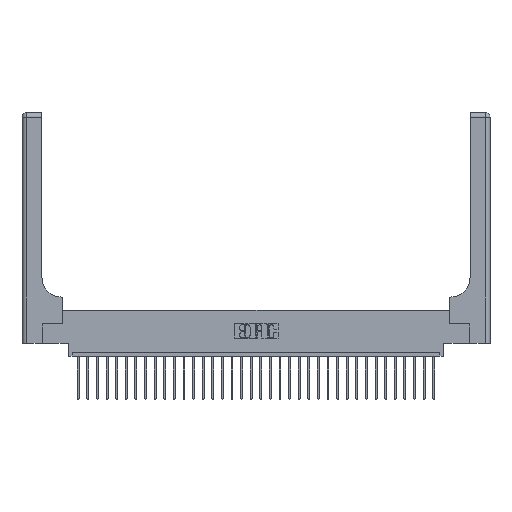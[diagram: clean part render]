
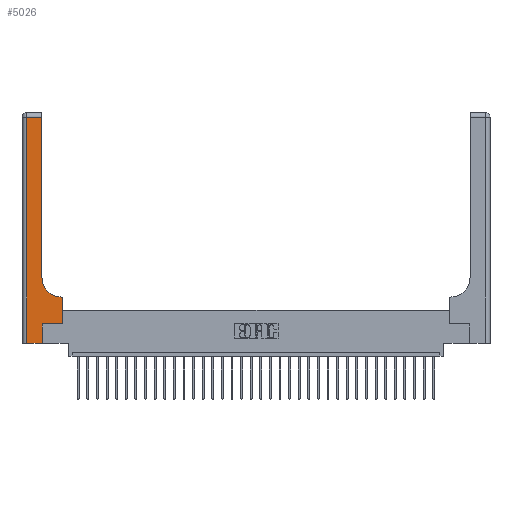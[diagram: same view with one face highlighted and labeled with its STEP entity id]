
A CAD part, top view. The second image highlights one B-rep face of the part: STEP entity #5026.
In plain terms, the highlighted planar face has unit normal (0, 0, 1).
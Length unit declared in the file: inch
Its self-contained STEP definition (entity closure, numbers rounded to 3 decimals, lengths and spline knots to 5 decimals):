
#54 = DIRECTION ( 'NONE',  ( -1., 0., 0. ) ) ;
#250 = CARTESIAN_POINT ( 'NONE',  ( 0.26, 2.94, 0.37 ) ) ;
#1270 = EDGE_LOOP ( 'NONE', ( #12998, #25585, #28772, #19783, #25614, #28763, #11897, #7678, #22462 ) ) ;
#1309 = DIRECTION ( 'NONE',  ( 0., -1., 0. ) ) ;
#1409 = EDGE_CURVE ( 'NONE', #23667, #22052, #14912, .T. ) ;
#2020 = VECTOR ( 'NONE', #9979, 39.37008 ) ;
#2103 = DIRECTION ( 'NONE',  ( 1., 0., 0. ) ) ;
#2382 = VECTOR ( 'NONE', #54, 39.37008 ) ;
#3548 = CIRCLE ( 'NONE', #27629, 0.25 ) ;
#3644 = VECTOR ( 'NONE', #27688, 39.37008 ) ;
#3798 = VECTOR ( 'NONE', #1309, 39.37008 ) ;
#4143 = VERTEX_POINT ( 'NONE', #25216 ) ;
#5026 = ADVANCED_FACE ( 'NONE', ( #11676 ), #18941, .F. ) ;
#5124 = DIRECTION ( 'NONE',  ( 0., 1., 0. ) ) ;
#6511 = DIRECTION ( 'NONE',  ( 1., 0., 0. ) ) ;
#7032 = VERTEX_POINT ( 'NONE', #24123 ) ;
#7678 = ORIENTED_EDGE ( 'NONE', *, *, #9285, .T. ) ;
#8913 = DIRECTION ( 'NONE',  ( 0., 0., -1. ) ) ;
#9285 = EDGE_CURVE ( 'NONE', #28783, #4143, #15762, .T. ) ;
#9369 = CARTESIAN_POINT ( 'NONE',  ( 0., 0., 0.37 ) ) ;
#9979 = DIRECTION ( 'NONE',  ( -1., 0., 0. ) ) ;
#10131 = VERTEX_POINT ( 'NONE', #18291 ) ;
#10431 = CARTESIAN_POINT ( 'NONE',  ( 0.528, 0.6, 0.37 ) ) ;
#10972 = VECTOR ( 'NONE', #6511, 39.37008 ) ;
#11676 = FACE_OUTER_BOUND ( 'NONE', #1270, .T. ) ;
#11800 = CARTESIAN_POINT ( 'NONE',  ( 0.06, 2.94, 0.37 ) ) ;
#11897 = ORIENTED_EDGE ( 'NONE', *, *, #12478, .T. ) ;
#12478 = EDGE_CURVE ( 'NONE', #27500, #28783, #18106, .T. ) ;
#12998 = ORIENTED_EDGE ( 'NONE', *, *, #15473, .T. ) ;
#14522 = CARTESIAN_POINT ( 'NONE',  ( 0.528, 0.25, 0.37 ) ) ;
#14668 = VECTOR ( 'NONE', #5124, 39.37008 ) ;
#14912 = LINE ( 'NONE', #20059, #3798 ) ;
#15473 = EDGE_CURVE ( 'NONE', #10131, #28225, #29435, .T. ) ;
#15762 = LINE ( 'NONE', #29845, #2382 ) ;
#15955 = EDGE_CURVE ( 'NONE', #4143, #10131, #3548, .T. ) ;
#16563 = VECTOR ( 'NONE', #22333, 39.37008 ) ;
#18106 = LINE ( 'NONE', #25066, #28516 ) ;
#18232 = CARTESIAN_POINT ( 'NONE',  ( 0.26, 3., 0.37 ) ) ;
#18291 = CARTESIAN_POINT ( 'NONE',  ( 0.26, 0.85, 0.37 ) ) ;
#18486 = CARTESIAN_POINT ( 'NONE',  ( 0., 3., 0.37 ) ) ;
#18571 = LINE ( 'NONE', #27647, #14668 ) ;
#18933 = VERTEX_POINT ( 'NONE', #20985 ) ;
#18941 = PLANE ( 'NONE',  #20073 ) ;
#19783 = ORIENTED_EDGE ( 'NONE', *, *, #28941, .T. ) ;
#20059 = CARTESIAN_POINT ( 'NONE',  ( 0.06, 3., 0.37 ) ) ;
#20073 = AXIS2_PLACEMENT_3D ( 'NONE', #18486, #28171, #27709 ) ;
#20985 = CARTESIAN_POINT ( 'NONE',  ( 0.265, 0.25, 0.37 ) ) ;
#21346 = EDGE_CURVE ( 'NONE', #28225, #23667, #24191, .T. ) ;
#22052 = VERTEX_POINT ( 'NONE', #28991 ) ;
#22333 = DIRECTION ( 'NONE',  ( 0., 1., 0. ) ) ;
#22462 = ORIENTED_EDGE ( 'NONE', *, *, #15955, .T. ) ;
#22979 = EDGE_CURVE ( 'NONE', #7032, #18933, #18571, .T. ) ;
#23174 = LINE ( 'NONE', #23764, #3644 ) ;
#23297 = LINE ( 'NONE', #9369, #10972 ) ;
#23667 = VERTEX_POINT ( 'NONE', #11800 ) ;
#23764 = CARTESIAN_POINT ( 'NONE',  ( 0.265, 0.25, 0.37 ) ) ;
#24123 = CARTESIAN_POINT ( 'NONE',  ( 0.265, 0., 0.37 ) ) ;
#24191 = LINE ( 'NONE', #26030, #2020 ) ;
#24964 = EDGE_CURVE ( 'NONE', #18933, #27500, #23174, .T. ) ;
#25066 = CARTESIAN_POINT ( 'NONE',  ( 0.528, 0.25, 0.37 ) ) ;
#25216 = CARTESIAN_POINT ( 'NONE',  ( 0.51, 0.6, 0.37 ) ) ;
#25585 = ORIENTED_EDGE ( 'NONE', *, *, #21346, .T. ) ;
#25614 = ORIENTED_EDGE ( 'NONE', *, *, #22979, .T. ) ;
#26030 = CARTESIAN_POINT ( 'NONE',  ( 0., 2.94, 0.37 ) ) ;
#27329 = DIRECTION ( 'NONE',  ( 0., 1., 0. ) ) ;
#27500 = VERTEX_POINT ( 'NONE', #14522 ) ;
#27629 = AXIS2_PLACEMENT_3D ( 'NONE', #27657, #8913, #2103 ) ;
#27647 = CARTESIAN_POINT ( 'NONE',  ( 0.265, 0., 0.37 ) ) ;
#27657 = CARTESIAN_POINT ( 'NONE',  ( 0.51, 0.85, 0.37 ) ) ;
#27688 = DIRECTION ( 'NONE',  ( 1., 0., 0. ) ) ;
#27709 = DIRECTION ( 'NONE',  ( -1., 0., 0. ) ) ;
#28171 = DIRECTION ( 'NONE',  ( 0., 0., -1. ) ) ;
#28225 = VERTEX_POINT ( 'NONE', #250 ) ;
#28516 = VECTOR ( 'NONE', #27329, 39.37008 ) ;
#28763 = ORIENTED_EDGE ( 'NONE', *, *, #24964, .T. ) ;
#28772 = ORIENTED_EDGE ( 'NONE', *, *, #1409, .T. ) ;
#28783 = VERTEX_POINT ( 'NONE', #10431 ) ;
#28941 = EDGE_CURVE ( 'NONE', #22052, #7032, #23297, .T. ) ;
#28991 = CARTESIAN_POINT ( 'NONE',  ( 0.06, 0., 0.37 ) ) ;
#29435 = LINE ( 'NONE', #18232, #16563 ) ;
#29845 = CARTESIAN_POINT ( 'NONE',  ( 0.26, 0.6, 0.37 ) ) ;
